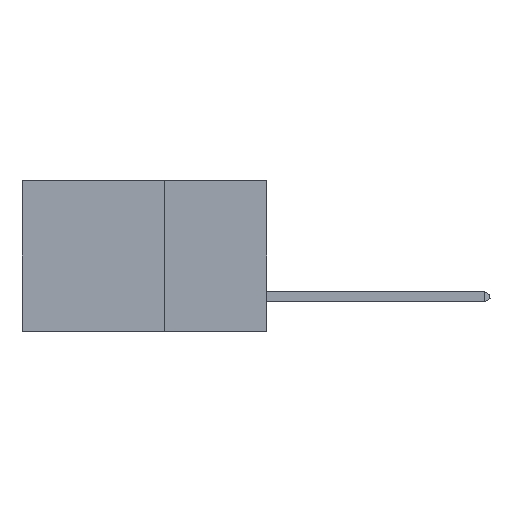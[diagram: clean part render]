
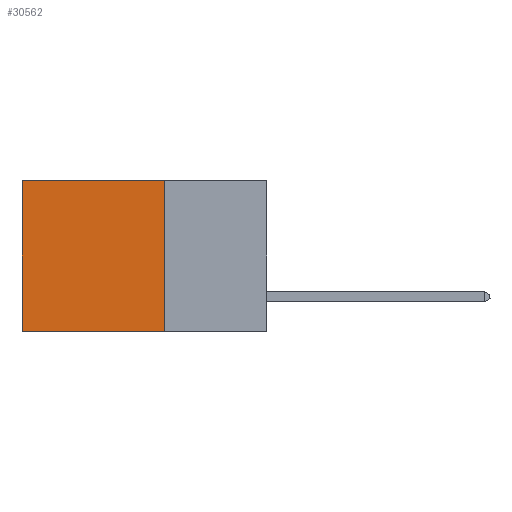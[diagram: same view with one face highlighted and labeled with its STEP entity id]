
A CAD part, left-side view. The second image highlights one B-rep face of the part: STEP entity #30562.
In plain terms, the highlighted planar face has unit normal (-1, 0, 0).
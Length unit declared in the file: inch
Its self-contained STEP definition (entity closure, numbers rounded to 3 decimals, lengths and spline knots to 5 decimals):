
#1260 = VECTOR ( 'NONE', #5750, 39.37008 ) ;
#2021 = ORIENTED_EDGE ( 'NONE', *, *, #27467, .F. ) ;
#2695 = DIRECTION ( 'NONE',  ( 0., 0., -1. ) ) ;
#3731 = VECTOR ( 'NONE', #2695, 39.37008 ) ;
#4782 = VECTOR ( 'NONE', #13848, 39.37008 ) ;
#5600 = CARTESIAN_POINT ( 'NONE',  ( 0.2875, 0.6, 0. ) ) ;
#5750 = DIRECTION ( 'NONE',  ( 0., 0., -1. ) ) ;
#6860 = VERTEX_POINT ( 'NONE', #15241 ) ;
#9842 = LINE ( 'NONE', #31213, #3731 ) ;
#11560 = CARTESIAN_POINT ( 'NONE',  ( 0.2875, 0.6, -0.37 ) ) ;
#13848 = DIRECTION ( 'NONE',  ( 0., 1., 0. ) ) ;
#15241 = CARTESIAN_POINT ( 'NONE',  ( 0.2875, 0.25, -0.37 ) ) ;
#15505 = VERTEX_POINT ( 'NONE', #21720 ) ;
#15714 = VERTEX_POINT ( 'NONE', #11560 ) ;
#17904 = EDGE_CURVE ( 'NONE', #28834, #15505, #23049, .T. ) ;
#18292 = EDGE_LOOP ( 'NONE', ( #41461, #24184, #2021, #39440 ) ) ;
#20548 = EDGE_CURVE ( 'NONE', #15505, #15714, #43257, .T. ) ;
#20593 = CARTESIAN_POINT ( 'NONE',  ( 0.2875, 0.25, 0. ) ) ;
#21720 = CARTESIAN_POINT ( 'NONE',  ( 0.2875, 0.6, 0. ) ) ;
#22546 = EDGE_CURVE ( 'NONE', #6860, #15714, #31928, .T. ) ;
#23049 = LINE ( 'NONE', #26978, #24161 ) ;
#24161 = VECTOR ( 'NONE', #31006, 39.37008 ) ;
#24184 = ORIENTED_EDGE ( 'NONE', *, *, #22546, .F. ) ;
#26978 = CARTESIAN_POINT ( 'NONE',  ( 0.2875, 0.25, 0. ) ) ;
#27467 = EDGE_CURVE ( 'NONE', #28834, #6860, #9842, .T. ) ;
#28568 = AXIS2_PLACEMENT_3D ( 'NONE', #20593, #38106, #30733 ) ;
#28834 = VERTEX_POINT ( 'NONE', #43217 ) ;
#30562 = ADVANCED_FACE ( 'NONE', ( #35049 ), #45138, .F. ) ;
#30733 = DIRECTION ( 'NONE',  ( 0., 0., -1. ) ) ;
#31006 = DIRECTION ( 'NONE',  ( 0., 1., 0. ) ) ;
#31213 = CARTESIAN_POINT ( 'NONE',  ( 0.2875, 0.25, 0. ) ) ;
#31928 = LINE ( 'NONE', #35208, #4782 ) ;
#35049 = FACE_OUTER_BOUND ( 'NONE', #18292, .T. ) ;
#35208 = CARTESIAN_POINT ( 'NONE',  ( 0.2875, 0.25, -0.37 ) ) ;
#38106 = DIRECTION ( 'NONE',  ( 1., 0., 0. ) ) ;
#39440 = ORIENTED_EDGE ( 'NONE', *, *, #17904, .T. ) ;
#41461 = ORIENTED_EDGE ( 'NONE', *, *, #20548, .T. ) ;
#43217 = CARTESIAN_POINT ( 'NONE',  ( 0.2875, 0.25, 0. ) ) ;
#43257 = LINE ( 'NONE', #5600, #1260 ) ;
#45138 = PLANE ( 'NONE',  #28568 ) ;
